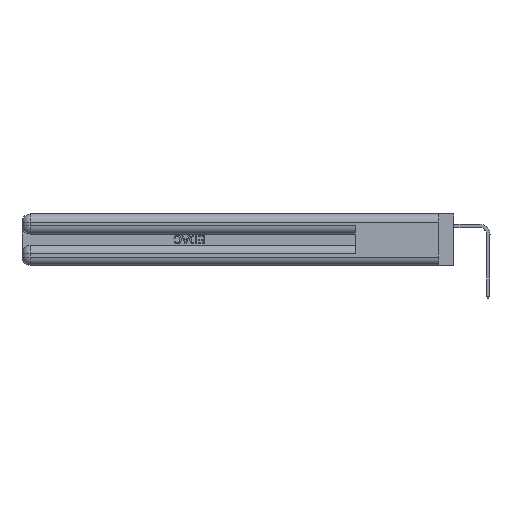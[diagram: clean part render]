
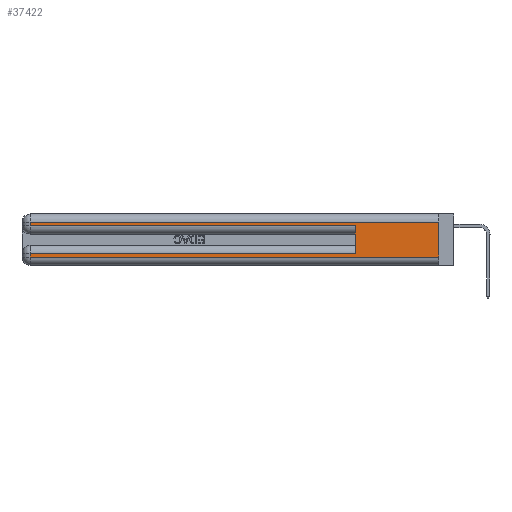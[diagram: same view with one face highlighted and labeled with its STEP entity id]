
A CAD part, left-side view. The second image highlights one B-rep face of the part: STEP entity #37422.
In plain terms, the highlighted planar face has unit normal (-1, 0, 0).
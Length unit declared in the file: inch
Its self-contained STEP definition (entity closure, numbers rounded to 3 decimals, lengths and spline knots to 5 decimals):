
#622 = ORIENTED_EDGE ( 'NONE', *, *, #9189, .F. ) ;
#1533 = CARTESIAN_POINT ( 'NONE',  ( 0., 0., 0.085 ) ) ;
#1751 = DIRECTION ( 'NONE',  ( 0., 0., -1. ) ) ;
#2016 = CARTESIAN_POINT ( 'NONE',  ( 0., 0., 0.31 ) ) ;
#3934 = CARTESIAN_POINT ( 'NONE',  ( 0., 2.94, 0.085 ) ) ;
#4180 = ORIENTED_EDGE ( 'NONE', *, *, #27858, .T. ) ;
#5110 = EDGE_CURVE ( 'NONE', #9022, #16077, #14694, .T. ) ;
#5305 = ORIENTED_EDGE ( 'NONE', *, *, #10784, .T. ) ;
#5383 = LINE ( 'NONE', #2016, #34244 ) ;
#6943 = CARTESIAN_POINT ( 'NONE',  ( 0., 0., 0.37 ) ) ;
#7436 = DIRECTION ( 'NONE',  ( 0., -1., 0. ) ) ;
#9022 = VERTEX_POINT ( 'NONE', #20201 ) ;
#9062 = VERTEX_POINT ( 'NONE', #31746 ) ;
#9149 = DIRECTION ( 'NONE',  ( 1., 0., 0. ) ) ;
#9189 = EDGE_CURVE ( 'NONE', #32083, #27432, #23057, .T. ) ;
#9592 = EDGE_LOOP ( 'NONE', ( #40632, #5305, #38888, #45937, #622, #4180, #39497, #24193 ) ) ;
#9960 = DIRECTION ( 'NONE',  ( 0., 0., 1. ) ) ;
#10553 = CARTESIAN_POINT ( 'NONE',  ( 0., 2.94, 0.285 ) ) ;
#10784 = EDGE_CURVE ( 'NONE', #9062, #47652, #5383, .T. ) ;
#13329 = EDGE_CURVE ( 'NONE', #9062, #16077, #29371, .T. ) ;
#14217 = VECTOR ( 'NONE', #9960, 39.37008 ) ;
#14246 = EDGE_CURVE ( 'NONE', #34277, #27432, #46878, .T. ) ;
#14635 = AXIS2_PLACEMENT_3D ( 'NONE', #24158, #9149, #35496 ) ;
#14694 = LINE ( 'NONE', #48705, #33561 ) ;
#15706 = LINE ( 'NONE', #46811, #44582 ) ;
#15915 = DIRECTION ( 'NONE',  ( 0., -1., 0. ) ) ;
#16077 = VERTEX_POINT ( 'NONE', #16673 ) ;
#16673 = CARTESIAN_POINT ( 'NONE',  ( 0., 0., 0.06 ) ) ;
#17235 = DIRECTION ( 'NONE',  ( 0., 0., -1. ) ) ;
#20171 = LINE ( 'NONE', #1533, #39031 ) ;
#20201 = CARTESIAN_POINT ( 'NONE',  ( 0., 2.94, 0.06 ) ) ;
#20632 = LINE ( 'NONE', #35994, #29509 ) ;
#23057 = LINE ( 'NONE', #32540, #14217 ) ;
#23326 = CARTESIAN_POINT ( 'NONE',  ( 0., 0., 0.285 ) ) ;
#24158 = CARTESIAN_POINT ( 'NONE',  ( 0., 0., 0.37 ) ) ;
#24193 = ORIENTED_EDGE ( 'NONE', *, *, #5110, .T. ) ;
#24561 = DIRECTION ( 'NONE',  ( 0., 1., 0. ) ) ;
#25316 = EDGE_CURVE ( 'NONE', #35049, #9022, #15706, .T. ) ;
#27432 = VERTEX_POINT ( 'NONE', #36618 ) ;
#27858 = EDGE_CURVE ( 'NONE', #32083, #35049, #20171, .T. ) ;
#27898 = DIRECTION ( 'NONE',  ( 0., 1., 0. ) ) ;
#29371 = LINE ( 'NONE', #6943, #48130 ) ;
#29509 = VECTOR ( 'NONE', #17235, 39.37008 ) ;
#31138 = FACE_OUTER_BOUND ( 'NONE', #9592, .T. ) ;
#31742 = PLANE ( 'NONE',  #14635 ) ;
#31746 = CARTESIAN_POINT ( 'NONE',  ( 0., 0., 0.31 ) ) ;
#31897 = CARTESIAN_POINT ( 'NONE',  ( 0., 0.6, 0.085 ) ) ;
#32083 = VERTEX_POINT ( 'NONE', #31897 ) ;
#32540 = CARTESIAN_POINT ( 'NONE',  ( 0., 0.6, 0.145 ) ) ;
#33561 = VECTOR ( 'NONE', #7436, 39.37008 ) ;
#34244 = VECTOR ( 'NONE', #24561, 39.37008 ) ;
#34277 = VERTEX_POINT ( 'NONE', #10553 ) ;
#35049 = VERTEX_POINT ( 'NONE', #3934 ) ;
#35496 = DIRECTION ( 'NONE',  ( 0., 0., -1. ) ) ;
#35994 = CARTESIAN_POINT ( 'NONE',  ( 0., 2.94, 0.37 ) ) ;
#36618 = CARTESIAN_POINT ( 'NONE',  ( 0., 0.6, 0.285 ) ) ;
#36894 = VECTOR ( 'NONE', #15915, 39.37008 ) ;
#37422 = ADVANCED_FACE ( 'NONE', ( #31138 ), #31742, .F. ) ;
#38888 = ORIENTED_EDGE ( 'NONE', *, *, #47031, .T. ) ;
#39031 = VECTOR ( 'NONE', #27898, 39.37008 ) ;
#39497 = ORIENTED_EDGE ( 'NONE', *, *, #25316, .T. ) ;
#40632 = ORIENTED_EDGE ( 'NONE', *, *, #13329, .F. ) ;
#40867 = DIRECTION ( 'NONE',  ( 0., 0., -1. ) ) ;
#44582 = VECTOR ( 'NONE', #1751, 39.37008 ) ;
#45937 = ORIENTED_EDGE ( 'NONE', *, *, #14246, .T. ) ;
#46811 = CARTESIAN_POINT ( 'NONE',  ( 0., 2.94, 0.37 ) ) ;
#46878 = LINE ( 'NONE', #23326, #36894 ) ;
#46936 = CARTESIAN_POINT ( 'NONE',  ( 0., 2.94, 0.31 ) ) ;
#47031 = EDGE_CURVE ( 'NONE', #47652, #34277, #20632, .T. ) ;
#47652 = VERTEX_POINT ( 'NONE', #46936 ) ;
#48130 = VECTOR ( 'NONE', #40867, 39.37008 ) ;
#48705 = CARTESIAN_POINT ( 'NONE',  ( 0., 0., 0.06 ) ) ;
